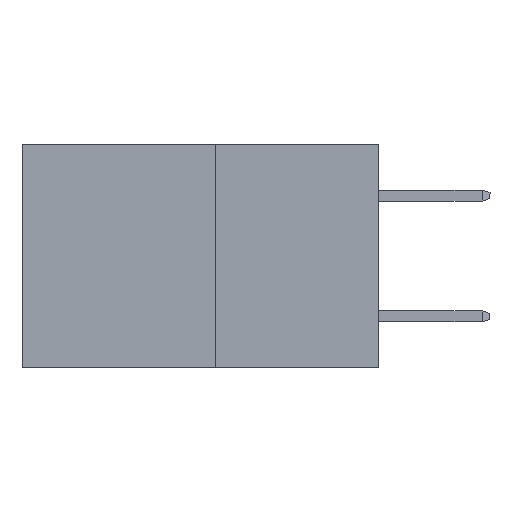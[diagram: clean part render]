
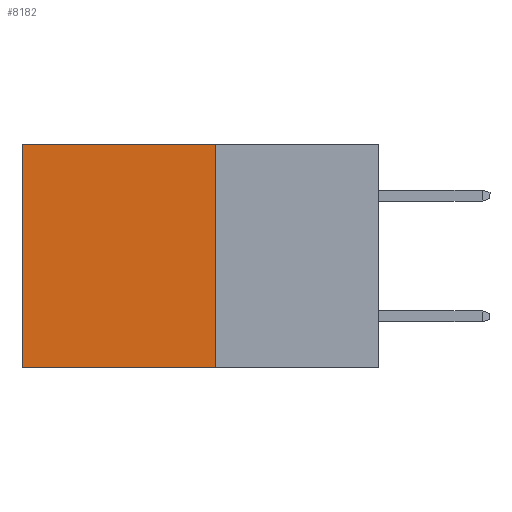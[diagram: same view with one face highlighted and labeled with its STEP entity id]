
A CAD part, left-side view. The second image highlights one B-rep face of the part: STEP entity #8182.
In plain terms, the highlighted planar face has unit normal (-1, 0, 0).
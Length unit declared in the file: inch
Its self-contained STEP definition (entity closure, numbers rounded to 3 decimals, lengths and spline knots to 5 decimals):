
#809 = VECTOR ( 'NONE', #1204, 39.37008 ) ;
#1204 = DIRECTION ( 'NONE',  ( 0., 0., -1. ) ) ;
#1226 = LINE ( 'NONE', #1295, #809 ) ;
#1267 = AXIS2_PLACEMENT_3D ( 'NONE', #2302, #2281, #2272 ) ;
#1295 = CARTESIAN_POINT ( 'NONE',  ( 0.277, 0.59, -0.37 ) ) ;
#1497 = VERTEX_POINT ( 'NONE', #7082 ) ;
#2174 = VERTEX_POINT ( 'NONE', #6616 ) ;
#2254 = ORIENTED_EDGE ( 'NONE', *, *, #6874, .T. ) ;
#2272 = DIRECTION ( 'NONE',  ( 0., 0., -1. ) ) ;
#2281 = DIRECTION ( 'NONE',  ( 1., 0., 0. ) ) ;
#2302 = CARTESIAN_POINT ( 'NONE',  ( 0.277, 0.27, -0.37 ) ) ;
#2322 = PLANE ( 'NONE',  #1267 ) ;
#2472 = ORIENTED_EDGE ( 'NONE', *, *, #8010, .F. ) ;
#2701 = ORIENTED_EDGE ( 'NONE', *, *, #3522, .T. ) ;
#3192 = CARTESIAN_POINT ( 'NONE',  ( 0.277, 0.27, -0.37 ) ) ;
#3222 = DIRECTION ( 'NONE',  ( 0., 0., -1. ) ) ;
#3464 = LINE ( 'NONE', #3192, #6919 ) ;
#3522 = EDGE_CURVE ( 'NONE', #1497, #5844, #3858, .T. ) ;
#3575 = CARTESIAN_POINT ( 'NONE',  ( 0.277, 0.27, 0. ) ) ;
#3583 = EDGE_CURVE ( 'NONE', #2174, #4753, #7292, .T. ) ;
#3662 = VECTOR ( 'NONE', #4164, 39.37008 ) ;
#3858 = LINE ( 'NONE', #3575, #3662 ) ;
#3977 = FACE_OUTER_BOUND ( 'NONE', #6907, .T. ) ;
#4047 = ORIENTED_EDGE ( 'NONE', *, *, #3583, .F. ) ;
#4164 = DIRECTION ( 'NONE',  ( 0., 1., 0. ) ) ;
#4753 = VERTEX_POINT ( 'NONE', #7872 ) ;
#5190 = VECTOR ( 'NONE', #5212, 39.37008 ) ;
#5212 = DIRECTION ( 'NONE',  ( 0., 1., 0. ) ) ;
#5383 = CARTESIAN_POINT ( 'NONE',  ( 0.277, 0.59, 0. ) ) ;
#5554 = CARTESIAN_POINT ( 'NONE',  ( 0.277, 0.27, -0.37 ) ) ;
#5844 = VERTEX_POINT ( 'NONE', #5383 ) ;
#6616 = CARTESIAN_POINT ( 'NONE',  ( 0.277, 0.27, -0.37 ) ) ;
#6874 = EDGE_CURVE ( 'NONE', #5844, #4753, #1226, .T. ) ;
#6907 = EDGE_LOOP ( 'NONE', ( #2254, #4047, #2472, #2701 ) ) ;
#6919 = VECTOR ( 'NONE', #3222, 39.37008 ) ;
#7082 = CARTESIAN_POINT ( 'NONE',  ( 0.277, 0.27, 0. ) ) ;
#7292 = LINE ( 'NONE', #5554, #5190 ) ;
#7872 = CARTESIAN_POINT ( 'NONE',  ( 0.277, 0.59, -0.37 ) ) ;
#8010 = EDGE_CURVE ( 'NONE', #1497, #2174, #3464, .T. ) ;
#8182 = ADVANCED_FACE ( 'NONE', ( #3977 ), #2322, .F. ) ;
